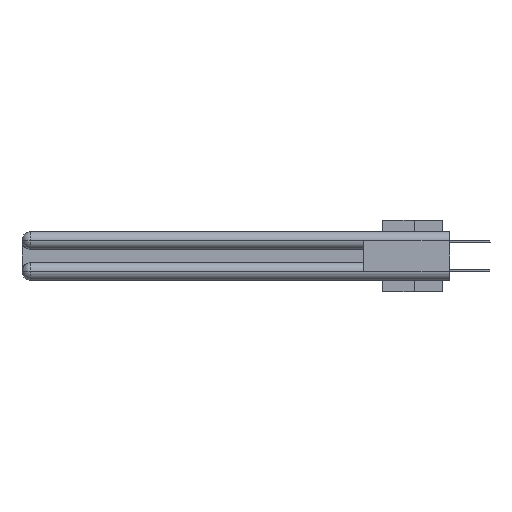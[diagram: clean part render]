
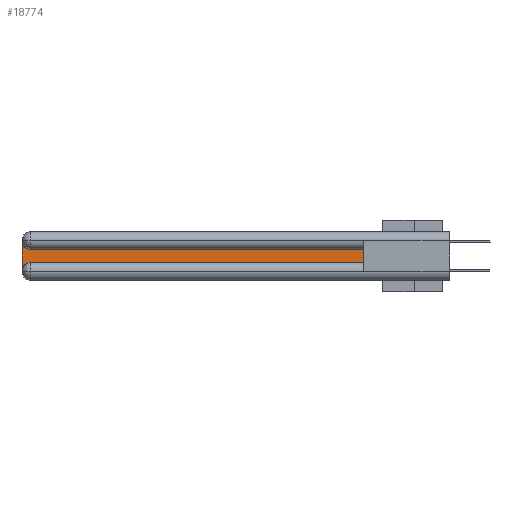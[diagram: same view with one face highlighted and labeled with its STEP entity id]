
A CAD part, left-side view. The second image highlights one B-rep face of the part: STEP entity #18774.
In plain terms, the highlighted planar face has unit normal (-1, 0, 0).
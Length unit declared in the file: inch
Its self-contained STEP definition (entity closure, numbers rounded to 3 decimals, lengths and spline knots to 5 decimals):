
#241 = VECTOR ( 'NONE', #969, 39.37008 ) ;
#969 = DIRECTION ( 'NONE',  ( 0., 1., 0. ) ) ;
#1319 = CARTESIAN_POINT ( 'NONE',  ( 0.075, 3., -0.1225 ) ) ;
#1804 = LINE ( 'NONE', #9481, #15188 ) ;
#3991 = CARTESIAN_POINT ( 'NONE',  ( 0.075, 2.94, -0.2775 ) ) ;
#4420 = EDGE_CURVE ( 'NONE', #25059, #14535, #1804, .T. ) ;
#5012 = AXIS2_PLACEMENT_3D ( 'NONE', #7535, #14325, #23464 ) ;
#5539 = CARTESIAN_POINT ( 'NONE',  ( 0.075, 2.94, -0.1225 ) ) ;
#5970 = EDGE_LOOP ( 'NONE', ( #24759, #25035, #16227, #7037, #29256, #7620 ) ) ;
#6418 = DIRECTION ( 'NONE',  ( 1., 0., 0. ) ) ;
#6689 = CARTESIAN_POINT ( 'NONE',  ( 0.075, 0.6, -0.1225 ) ) ;
#7037 = ORIENTED_EDGE ( 'NONE', *, *, #7733, .T. ) ;
#7466 = VERTEX_POINT ( 'NONE', #12083 ) ;
#7535 = CARTESIAN_POINT ( 'NONE',  ( 0.075, 2.94, -0.0625 ) ) ;
#7620 = ORIENTED_EDGE ( 'NONE', *, *, #24431, .T. ) ;
#7733 = EDGE_CURVE ( 'NONE', #14535, #7466, #26352, .T. ) ;
#9481 = CARTESIAN_POINT ( 'NONE',  ( 0.075, 3., -0.2175 ) ) ;
#9977 = VECTOR ( 'NONE', #10961, 39.37008 ) ;
#10004 = EDGE_CURVE ( 'NONE', #19913, #25059, #27698, .T. ) ;
#10936 = EDGE_CURVE ( 'NONE', #24751, #19913, #16547, .T. ) ;
#10961 = DIRECTION ( 'NONE',  ( 0., -1., 0. ) ) ;
#11042 = EDGE_CURVE ( 'NONE', #7466, #24075, #23082, .T. ) ;
#11829 = CARTESIAN_POINT ( 'NONE',  ( 0.075, 3., -0.0625 ) ) ;
#12083 = CARTESIAN_POINT ( 'NONE',  ( 0.075, 2.94, -0.2175 ) ) ;
#12564 = CARTESIAN_POINT ( 'NONE',  ( 0.075, 0.6, -0.2175 ) ) ;
#13472 = VECTOR ( 'NONE', #19680, 39.37008 ) ;
#13835 = CARTESIAN_POINT ( 'NONE',  ( 0.075, 0.6, -0.1225 ) ) ;
#14179 = FACE_OUTER_BOUND ( 'NONE', #5970, .T. ) ;
#14325 = DIRECTION ( 'NONE',  ( 1., 0., 0. ) ) ;
#14535 = VERTEX_POINT ( 'NONE', #16628 ) ;
#15188 = VECTOR ( 'NONE', #16707, 39.37008 ) ;
#15742 = CARTESIAN_POINT ( 'NONE',  ( 0.075, 0.6, -0.2175 ) ) ;
#16227 = ORIENTED_EDGE ( 'NONE', *, *, #4420, .T. ) ;
#16547 = LINE ( 'NONE', #13835, #241 ) ;
#16628 = CARTESIAN_POINT ( 'NONE',  ( 0.075, 3., -0.2775 ) ) ;
#16707 = DIRECTION ( 'NONE',  ( 0., 0., -1. ) ) ;
#18774 = ADVANCED_FACE ( 'NONE', ( #14179 ), #24429, .F. ) ;
#19680 = DIRECTION ( 'NONE',  ( 0., 0., 1. ) ) ;
#19859 = DIRECTION ( 'NONE',  ( 1., 0., 0. ) ) ;
#19913 = VERTEX_POINT ( 'NONE', #5539 ) ;
#21846 = LINE ( 'NONE', #12564, #13472 ) ;
#23082 = LINE ( 'NONE', #27093, #9977 ) ;
#23464 = DIRECTION ( 'NONE',  ( 0., 0., -1. ) ) ;
#24075 = VERTEX_POINT ( 'NONE', #15742 ) ;
#24418 = AXIS2_PLACEMENT_3D ( 'NONE', #1319, #19859, #28982 ) ;
#24429 = PLANE ( 'NONE',  #24418 ) ;
#24431 = EDGE_CURVE ( 'NONE', #24075, #24751, #21846, .T. ) ;
#24751 = VERTEX_POINT ( 'NONE', #6689 ) ;
#24759 = ORIENTED_EDGE ( 'NONE', *, *, #10936, .T. ) ;
#25035 = ORIENTED_EDGE ( 'NONE', *, *, #10004, .T. ) ;
#25059 = VERTEX_POINT ( 'NONE', #11829 ) ;
#26352 = CIRCLE ( 'NONE', #28665, 0.06 ) ;
#26980 = DIRECTION ( 'NONE',  ( 0., 0., -1. ) ) ;
#27093 = CARTESIAN_POINT ( 'NONE',  ( 0.075, 0.6, -0.2175 ) ) ;
#27698 = CIRCLE ( 'NONE', #5012, 0.06 ) ;
#28665 = AXIS2_PLACEMENT_3D ( 'NONE', #3991, #6418, #26980 ) ;
#28982 = DIRECTION ( 'NONE',  ( 0., 0., -1. ) ) ;
#29256 = ORIENTED_EDGE ( 'NONE', *, *, #11042, .T. ) ;
